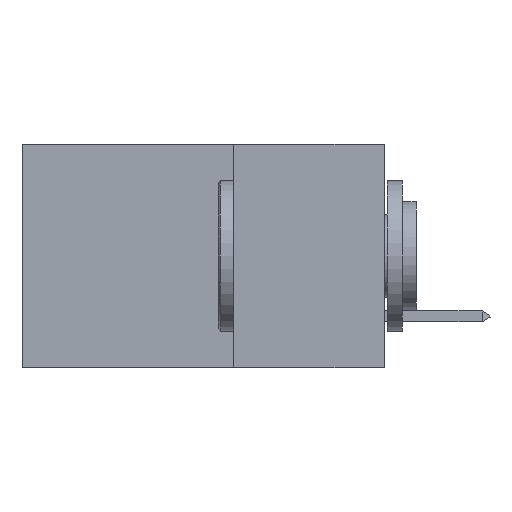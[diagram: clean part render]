
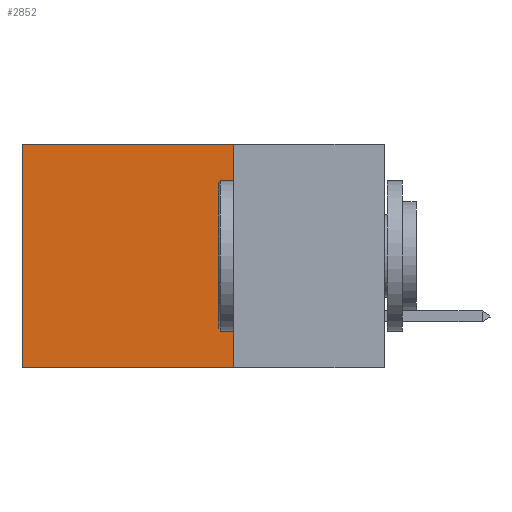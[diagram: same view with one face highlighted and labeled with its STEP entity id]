
A CAD part, left-side view. The second image highlights one B-rep face of the part: STEP entity #2852.
In plain terms, the highlighted planar face has unit normal (-1, 0, 0).
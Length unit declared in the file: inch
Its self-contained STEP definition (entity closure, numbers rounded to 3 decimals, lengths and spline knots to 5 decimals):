
#106 = EDGE_CURVE ( 'NONE', #979, #8714, #1573, .T. ) ;
#243 = DIRECTION ( 'NONE',  ( 1., 0., 0. ) ) ;
#357 = DIRECTION ( 'NONE',  ( 0., 0., -1. ) ) ;
#424 = CARTESIAN_POINT ( 'NONE',  ( 0.2875, 0.6, -0.37 ) ) ;
#979 = VERTEX_POINT ( 'NONE', #8863 ) ;
#1147 = ORIENTED_EDGE ( 'NONE', *, *, #9475, .F. ) ;
#1172 = LINE ( 'NONE', #9728, #3632 ) ;
#1380 = CARTESIAN_POINT ( 'NONE',  ( 0.2875, 0.25, 0. ) ) ;
#1458 = DIRECTION ( 'NONE',  ( 0., 0., -1. ) ) ;
#1573 = LINE ( 'NONE', #1380, #3290 ) ;
#1782 = DIRECTION ( 'NONE',  ( 0., 0., -1. ) ) ;
#2115 = AXIS2_PLACEMENT_3D ( 'NONE', #8057, #243, #1782 ) ;
#2435 = EDGE_CURVE ( 'NONE', #6634, #9024, #4328, .T. ) ;
#2852 = ADVANCED_FACE ( 'NONE', ( #3133 ), #7246, .F. ) ;
#2885 = CARTESIAN_POINT ( 'NONE',  ( 0.2875, 0.25, -0.37 ) ) ;
#3064 = ORIENTED_EDGE ( 'NONE', *, *, #3621, .T. ) ;
#3133 = FACE_OUTER_BOUND ( 'NONE', #4196, .T. ) ;
#3290 = VECTOR ( 'NONE', #7691, 39.37008 ) ;
#3621 = EDGE_CURVE ( 'NONE', #8714, #9024, #1172, .T. ) ;
#3632 = VECTOR ( 'NONE', #357, 39.37008 ) ;
#3936 = CARTESIAN_POINT ( 'NONE',  ( 0.2875, 0.25, -0.37 ) ) ;
#4067 = CARTESIAN_POINT ( 'NONE',  ( 0.2875, 0.6, 0. ) ) ;
#4196 = EDGE_LOOP ( 'NONE', ( #3064, #6171, #1147, #5744 ) ) ;
#4328 = LINE ( 'NONE', #2885, #8272 ) ;
#5744 = ORIENTED_EDGE ( 'NONE', *, *, #106, .T. ) ;
#6171 = ORIENTED_EDGE ( 'NONE', *, *, #2435, .F. ) ;
#6634 = VERTEX_POINT ( 'NONE', #3936 ) ;
#7246 = PLANE ( 'NONE',  #2115 ) ;
#7683 = DIRECTION ( 'NONE',  ( 0., 1., 0. ) ) ;
#7691 = DIRECTION ( 'NONE',  ( 0., 1., 0. ) ) ;
#7779 = LINE ( 'NONE', #9918, #9970 ) ;
#8057 = CARTESIAN_POINT ( 'NONE',  ( 0.2875, 0.25, 0. ) ) ;
#8272 = VECTOR ( 'NONE', #7683, 39.37008 ) ;
#8714 = VERTEX_POINT ( 'NONE', #4067 ) ;
#8863 = CARTESIAN_POINT ( 'NONE',  ( 0.2875, 0.25, 0. ) ) ;
#9024 = VERTEX_POINT ( 'NONE', #424 ) ;
#9475 = EDGE_CURVE ( 'NONE', #979, #6634, #7779, .T. ) ;
#9728 = CARTESIAN_POINT ( 'NONE',  ( 0.2875, 0.6, 0. ) ) ;
#9918 = CARTESIAN_POINT ( 'NONE',  ( 0.2875, 0.25, 0. ) ) ;
#9970 = VECTOR ( 'NONE', #1458, 39.37008 ) ;
